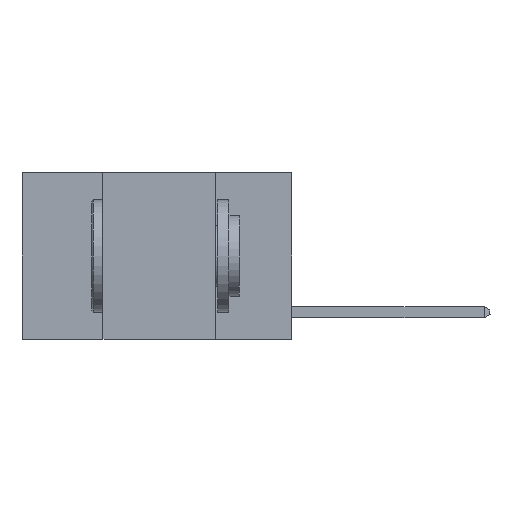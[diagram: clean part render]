
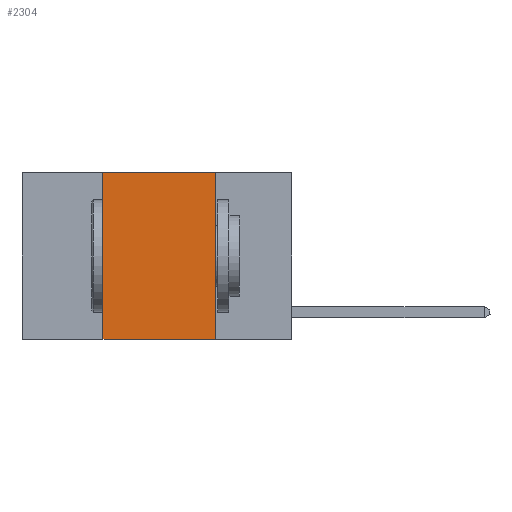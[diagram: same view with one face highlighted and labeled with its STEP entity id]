
A CAD part, left-side view. The second image highlights one B-rep face of the part: STEP entity #2304.
In plain terms, the highlighted planar face has unit normal (-1, 0, 0).
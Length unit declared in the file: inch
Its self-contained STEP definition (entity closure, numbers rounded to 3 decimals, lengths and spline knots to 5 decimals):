
#84 = VECTOR ( 'NONE', #22178, 39.37008 ) ;
#444 = CARTESIAN_POINT ( 'NONE',  ( 0., 0.17, 0. ) ) ;
#630 = DIRECTION ( 'NONE',  ( 0., -1., 0. ) ) ;
#1536 = CARTESIAN_POINT ( 'NONE',  ( 0., 0.42, 0. ) ) ;
#1563 = CARTESIAN_POINT ( 'NONE',  ( 0., 0.6, 0. ) ) ;
#2304 = ADVANCED_FACE ( 'NONE', ( #7625 ), #4117, .F. ) ;
#2476 = ORIENTED_EDGE ( 'NONE', *, *, #13220, .F. ) ;
#3443 = DIRECTION ( 'NONE',  ( 0., -1., 0. ) ) ;
#3467 = LINE ( 'NONE', #1563, #12598 ) ;
#3769 = ORIENTED_EDGE ( 'NONE', *, *, #21550, .T. ) ;
#4117 = PLANE ( 'NONE',  #9813 ) ;
#5335 = CARTESIAN_POINT ( 'NONE',  ( 0., 0.42, -0.37 ) ) ;
#7625 = FACE_OUTER_BOUND ( 'NONE', #16773, .T. ) ;
#8858 = VERTEX_POINT ( 'NONE', #5335 ) ;
#9691 = VECTOR ( 'NONE', #17590, 39.37008 ) ;
#9813 = AXIS2_PLACEMENT_3D ( 'NONE', #15555, #11749, #17206 ) ;
#11749 = DIRECTION ( 'NONE',  ( 1., 0., 0. ) ) ;
#12256 = ORIENTED_EDGE ( 'NONE', *, *, #13489, .F. ) ;
#12598 = VECTOR ( 'NONE', #3443, 39.37008 ) ;
#12670 = CARTESIAN_POINT ( 'NONE',  ( 0., 0.17, -0.37 ) ) ;
#13220 = EDGE_CURVE ( 'NONE', #20606, #20808, #19323, .T. ) ;
#13489 = EDGE_CURVE ( 'NONE', #8858, #23354, #22400, .T. ) ;
#13697 = CARTESIAN_POINT ( 'NONE',  ( 0., 0.17, 0. ) ) ;
#14469 = CARTESIAN_POINT ( 'NONE',  ( 0., 0.42, 0. ) ) ;
#15420 = VECTOR ( 'NONE', #630, 39.37008 ) ;
#15555 = CARTESIAN_POINT ( 'NONE',  ( 0., 0.6, 0. ) ) ;
#16773 = EDGE_LOOP ( 'NONE', ( #2476, #17936, #12256, #3769 ) ) ;
#17206 = DIRECTION ( 'NONE',  ( 0., 0., -1. ) ) ;
#17590 = DIRECTION ( 'NONE',  ( 0., 0., -1. ) ) ;
#17899 = CARTESIAN_POINT ( 'NONE',  ( 0., 0.6, -0.37 ) ) ;
#17936 = ORIENTED_EDGE ( 'NONE', *, *, #23353, .F. ) ;
#19323 = LINE ( 'NONE', #444, #9691 ) ;
#19753 = LINE ( 'NONE', #17899, #15420 ) ;
#20606 = VERTEX_POINT ( 'NONE', #13697 ) ;
#20808 = VERTEX_POINT ( 'NONE', #12670 ) ;
#21550 = EDGE_CURVE ( 'NONE', #8858, #20808, #19753, .T. ) ;
#22178 = DIRECTION ( 'NONE',  ( 0., 0., 1. ) ) ;
#22400 = LINE ( 'NONE', #14469, #84 ) ;
#23353 = EDGE_CURVE ( 'NONE', #23354, #20606, #3467, .T. ) ;
#23354 = VERTEX_POINT ( 'NONE', #1536 ) ;
